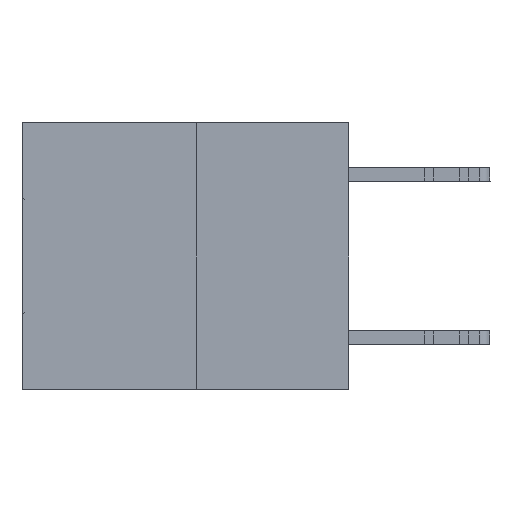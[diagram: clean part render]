
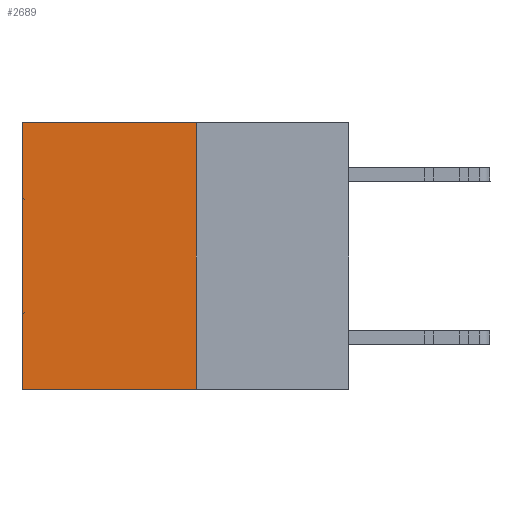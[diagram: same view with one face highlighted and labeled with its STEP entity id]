
A CAD part, left-side view. The second image highlights one B-rep face of the part: STEP entity #2689.
In plain terms, the highlighted planar face has unit normal (-1, 0, 0).
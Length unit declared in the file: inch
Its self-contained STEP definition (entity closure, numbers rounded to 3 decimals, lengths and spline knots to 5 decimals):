
#2689 = ADVANCED_FACE ( 'NONE', ( #17879 ), #29983, .F. ) ;
#3219 = CARTESIAN_POINT ( 'NONE',  ( 0.3165, 0.28, -0.49 ) ) ;
#3231 = VECTOR ( 'NONE', #23666, 39.37008 ) ;
#3309 = ORIENTED_EDGE ( 'NONE', *, *, #29036, .T. ) ;
#3962 = ORIENTED_EDGE ( 'NONE', *, *, #6193, .T. ) ;
#4183 = LINE ( 'NONE', #4480, #5418 ) ;
#4480 = CARTESIAN_POINT ( 'NONE',  ( 0.3165, 0.28, -0.49 ) ) ;
#5243 = EDGE_CURVE ( 'NONE', #9546, #22600, #4183, .T. ) ;
#5418 = VECTOR ( 'NONE', #18796, 39.37008 ) ;
#6193 = EDGE_CURVE ( 'NONE', #32111, #31080, #27163, .T. ) ;
#7158 = VECTOR ( 'NONE', #16531, 39.37008 ) ;
#7285 = LINE ( 'NONE', #3219, #3231 ) ;
#8036 = CARTESIAN_POINT ( 'NONE',  ( 0.3165, 0.28, 0. ) ) ;
#9449 = EDGE_LOOP ( 'NONE', ( #3962, #28470, #32554, #3309 ) ) ;
#9546 = VERTEX_POINT ( 'NONE', #18061 ) ;
#9709 = CARTESIAN_POINT ( 'NONE',  ( 0.3165, 0.28, -0.49 ) ) ;
#10592 = AXIS2_PLACEMENT_3D ( 'NONE', #9709, #17642, #12567 ) ;
#11915 = LINE ( 'NONE', #8036, #7158 ) ;
#12567 = DIRECTION ( 'NONE',  ( 0., 0., -1. ) ) ;
#13322 = CARTESIAN_POINT ( 'NONE',  ( 0.3165, 0.6, -0.49 ) ) ;
#16531 = DIRECTION ( 'NONE',  ( 0., 1., 0. ) ) ;
#17642 = DIRECTION ( 'NONE',  ( 1., 0., 0. ) ) ;
#17879 = FACE_OUTER_BOUND ( 'NONE', #9449, .T. ) ;
#18061 = CARTESIAN_POINT ( 'NONE',  ( 0.3165, 0.28, 0. ) ) ;
#18796 = DIRECTION ( 'NONE',  ( 0., 0., -1. ) ) ;
#21398 = EDGE_CURVE ( 'NONE', #22600, #31080, #7285, .T. ) ;
#22600 = VERTEX_POINT ( 'NONE', #24118 ) ;
#23666 = DIRECTION ( 'NONE',  ( 0., 1., 0. ) ) ;
#24118 = CARTESIAN_POINT ( 'NONE',  ( 0.3165, 0.28, -0.49 ) ) ;
#24755 = VECTOR ( 'NONE', #26057, 39.37008 ) ;
#26057 = DIRECTION ( 'NONE',  ( 0., 0., -1. ) ) ;
#27163 = LINE ( 'NONE', #31057, #24755 ) ;
#28470 = ORIENTED_EDGE ( 'NONE', *, *, #21398, .F. ) ;
#29036 = EDGE_CURVE ( 'NONE', #9546, #32111, #11915, .T. ) ;
#29983 = PLANE ( 'NONE',  #10592 ) ;
#31042 = CARTESIAN_POINT ( 'NONE',  ( 0.3165, 0.6, 0. ) ) ;
#31057 = CARTESIAN_POINT ( 'NONE',  ( 0.3165, 0.6, -0.49 ) ) ;
#31080 = VERTEX_POINT ( 'NONE', #13322 ) ;
#32111 = VERTEX_POINT ( 'NONE', #31042 ) ;
#32554 = ORIENTED_EDGE ( 'NONE', *, *, #5243, .F. ) ;
